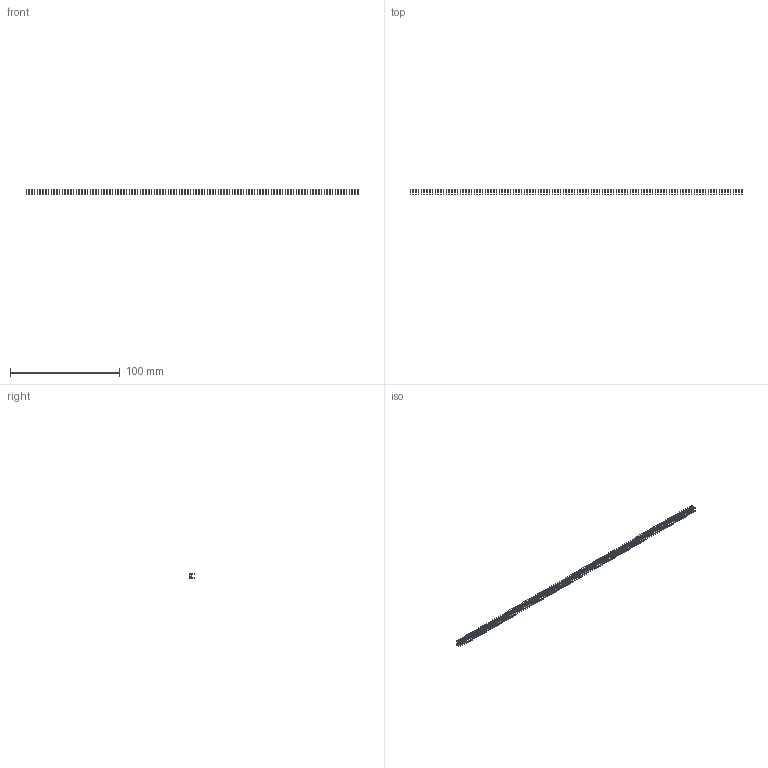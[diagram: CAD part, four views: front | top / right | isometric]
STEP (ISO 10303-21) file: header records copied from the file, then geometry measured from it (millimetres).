
FILE_DESCRIPTION (( 'STEP AP203' ), '1' );
FILE_NAME ('105-120-208-100.STEP', '2020-04-08T01:27:42', ( '' ), ( '' ), 'SwSTEP 2.0', 'SolidWorks 2016', '' );
FILE_SCHEMA (( 'CONFIG_CONTROL_DESIGN' ));
Length unit declared in the file: inch
Products named in the file (2): 100-290-001_100-290-208; 105-120-208-100
Assembly tree (120 placements, depth 2):
  105-120-208-100
    100-290-001_100-290-208  x120
Bounding box: 302.77 x 4.83 x 5.17 mm (x, y, z)
Volume: 825.7 mm3; surface area: 5099.5 mm2
Topology: 120 solids, 120 shells, 3000 faces, 8280 edges, 5520 vertices
Faces by surface type: plane 2640, cylinder 360
Entity records: 4797 total; most frequent: DIRECTION 371, CARTESIAN_POINT 263, LOCAL_TIME 250, COORDINATED_UNIVERSAL_TIME_OFFSET 250, CALENDAR_DATE 250, DATE_AND_TIME 250, AXIS2_PLACEMENT_3D 154, ORIENTED_EDGE 138
